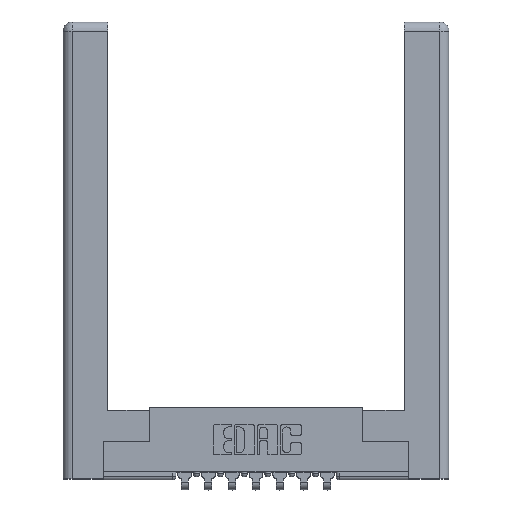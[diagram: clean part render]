
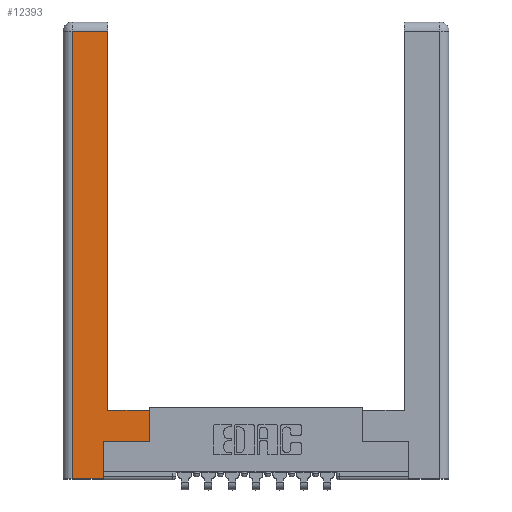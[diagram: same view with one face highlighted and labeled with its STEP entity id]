
A CAD part, top view. The second image highlights one B-rep face of the part: STEP entity #12393.
In plain terms, the highlighted planar face has unit normal (0, 0, 1).
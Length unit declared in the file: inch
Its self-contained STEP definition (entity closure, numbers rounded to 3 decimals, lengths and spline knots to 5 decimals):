
#359 = VECTOR ( 'NONE', #10221, 39.37008 ) ;
#908 = CARTESIAN_POINT ( 'NONE',  ( 0., 0., 0. ) ) ;
#1361 = CARTESIAN_POINT ( 'NONE',  ( 0.265, 0.245, 0. ) ) ;
#1560 = ORIENTED_EDGE ( 'NONE', *, *, #12342, .T. ) ;
#1591 = LINE ( 'NONE', #12900, #4740 ) ;
#1841 = CARTESIAN_POINT ( 'NONE',  ( 0.265, 0., 0. ) ) ;
#1851 = VECTOR ( 'NONE', #4665, 39.37008 ) ;
#2638 = LINE ( 'NONE', #9746, #12424 ) ;
#2761 = DIRECTION ( 'NONE',  ( 0., 1., 0. ) ) ;
#2871 = LINE ( 'NONE', #7850, #8138 ) ;
#2882 = PLANE ( 'NONE',  #3596 ) ;
#3190 = CARTESIAN_POINT ( 'NONE',  ( 0.0615, 0., 0. ) ) ;
#3434 = ORIENTED_EDGE ( 'NONE', *, *, #6350, .T. ) ;
#3452 = EDGE_CURVE ( 'NONE', #9753, #12649, #2871, .T. ) ;
#3596 = AXIS2_PLACEMENT_3D ( 'NONE', #908, #7863, #9012 ) ;
#3780 = CARTESIAN_POINT ( 'NONE',  ( 0.265, 0., 0. ) ) ;
#3806 = FACE_OUTER_BOUND ( 'NONE', #10149, .T. ) ;
#3812 = VERTEX_POINT ( 'NONE', #3780 ) ;
#3961 = CARTESIAN_POINT ( 'NONE',  ( 0.565, 0.245, 0. ) ) ;
#3962 = VERTEX_POINT ( 'NONE', #4174 ) ;
#4174 = CARTESIAN_POINT ( 'NONE',  ( 0.0615, 0., 0. ) ) ;
#4260 = CARTESIAN_POINT ( 'NONE',  ( 0.295, 0.45, 0. ) ) ;
#4581 = ORIENTED_EDGE ( 'NONE', *, *, #4699, .T. ) ;
#4665 = DIRECTION ( 'NONE',  ( -1., 0., 0. ) ) ;
#4699 = EDGE_CURVE ( 'NONE', #3812, #4860, #1591, .T. ) ;
#4740 = VECTOR ( 'NONE', #2761, 39.37008 ) ;
#4808 = LINE ( 'NONE', #3961, #8871 ) ;
#4860 = VERTEX_POINT ( 'NONE', #1361 ) ;
#4864 = CARTESIAN_POINT ( 'NONE',  ( 0.295, 2.94, 0. ) ) ;
#5034 = ORIENTED_EDGE ( 'NONE', *, *, #8078, .T. ) ;
#5094 = ORIENTED_EDGE ( 'NONE', *, *, #8901, .T. ) ;
#5231 = VECTOR ( 'NONE', #8164, 39.37008 ) ;
#5673 = DIRECTION ( 'NONE',  ( 0., 1., 0. ) ) ;
#5891 = CARTESIAN_POINT ( 'NONE',  ( 0.565, 0.45, 0. ) ) ;
#6171 = LINE ( 'NONE', #3190, #359 ) ;
#6350 = EDGE_CURVE ( 'NONE', #9356, #11076, #7334, .T. ) ;
#7017 = ORIENTED_EDGE ( 'NONE', *, *, #7466, .T. ) ;
#7059 = LINE ( 'NONE', #1841, #10585 ) ;
#7334 = LINE ( 'NONE', #8602, #1851 ) ;
#7466 = EDGE_CURVE ( 'NONE', #12649, #3962, #6171, .T. ) ;
#7850 = CARTESIAN_POINT ( 'NONE',  ( 0.0615, 2.94, 0. ) ) ;
#7863 = DIRECTION ( 'NONE',  ( 0., 0., -1. ) ) ;
#8013 = DIRECTION ( 'NONE',  ( 1., 0., 0. ) ) ;
#8078 = EDGE_CURVE ( 'NONE', #11076, #9753, #2638, .T. ) ;
#8138 = VECTOR ( 'NONE', #11900, 39.37008 ) ;
#8164 = DIRECTION ( 'NONE',  ( 0., 1., 0. ) ) ;
#8602 = CARTESIAN_POINT ( 'NONE',  ( 0.295, 0.45, 0. ) ) ;
#8806 = VERTEX_POINT ( 'NONE', #12596 ) ;
#8871 = VECTOR ( 'NONE', #8013, 39.37008 ) ;
#8901 = EDGE_CURVE ( 'NONE', #8806, #9356, #9107, .T. ) ;
#9012 = DIRECTION ( 'NONE',  ( -1., 0., 0. ) ) ;
#9107 = LINE ( 'NONE', #5891, #5231 ) ;
#9342 = EDGE_CURVE ( 'NONE', #4860, #8806, #4808, .T. ) ;
#9356 = VERTEX_POINT ( 'NONE', #12126 ) ;
#9716 = CARTESIAN_POINT ( 'NONE',  ( 0.0615, 2.94, 0. ) ) ;
#9746 = CARTESIAN_POINT ( 'NONE',  ( 0.295, 3., 0. ) ) ;
#9753 = VERTEX_POINT ( 'NONE', #4864 ) ;
#10149 = EDGE_LOOP ( 'NONE', ( #5034, #12371, #7017, #1560, #4581, #12809, #5094, #3434 ) ) ;
#10221 = DIRECTION ( 'NONE',  ( 0., -1., 0. ) ) ;
#10585 = VECTOR ( 'NONE', #11184, 39.37008 ) ;
#11076 = VERTEX_POINT ( 'NONE', #4260 ) ;
#11184 = DIRECTION ( 'NONE',  ( 1., 0., 0. ) ) ;
#11900 = DIRECTION ( 'NONE',  ( -1., 0., 0. ) ) ;
#12126 = CARTESIAN_POINT ( 'NONE',  ( 0.565, 0.45, 0. ) ) ;
#12342 = EDGE_CURVE ( 'NONE', #3962, #3812, #7059, .T. ) ;
#12371 = ORIENTED_EDGE ( 'NONE', *, *, #3452, .T. ) ;
#12393 = ADVANCED_FACE ( 'NONE', ( #3806 ), #2882, .F. ) ;
#12424 = VECTOR ( 'NONE', #5673, 39.37008 ) ;
#12596 = CARTESIAN_POINT ( 'NONE',  ( 0.565, 0.245, 0. ) ) ;
#12649 = VERTEX_POINT ( 'NONE', #9716 ) ;
#12809 = ORIENTED_EDGE ( 'NONE', *, *, #9342, .T. ) ;
#12900 = CARTESIAN_POINT ( 'NONE',  ( 0.265, 0.245, 0. ) ) ;
